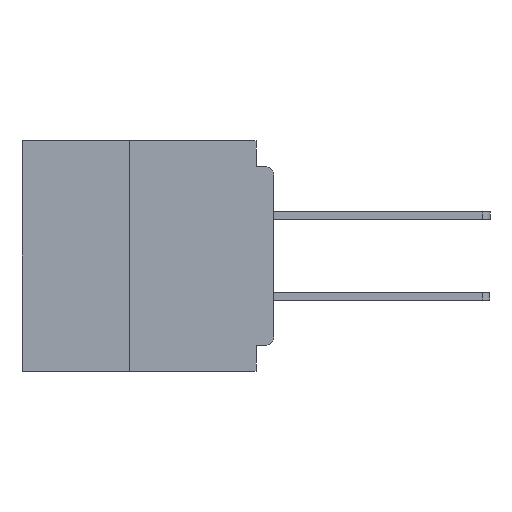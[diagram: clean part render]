
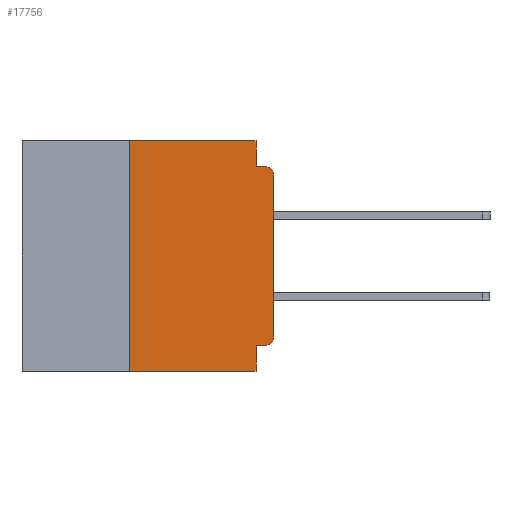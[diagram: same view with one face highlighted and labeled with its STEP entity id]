
A CAD part, left-side view. The second image highlights one B-rep face of the part: STEP entity #17756.
In plain terms, the highlighted planar face has unit normal (-1, 0, 0).
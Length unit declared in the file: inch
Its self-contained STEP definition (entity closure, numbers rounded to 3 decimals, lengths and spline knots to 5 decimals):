
#354 = DIRECTION ( 'NONE',  ( 0., 0., -1. ) ) ;
#1118 = EDGE_CURVE ( 'NONE', #3465, #8036, #11682, .T. ) ;
#2225 = CARTESIAN_POINT ( 'NONE',  ( 0., 0., -0.06 ) ) ;
#2336 = CARTESIAN_POINT ( 'NONE',  ( 0., 0.015, -0.355 ) ) ;
#2476 = EDGE_LOOP ( 'NONE', ( #45321, #27061, #30065, #25355, #29021, #8295, #48030, #5185, #6686, #10354 ) ) ;
#3120 = AXIS2_PLACEMENT_3D ( 'NONE', #16670, #45256, #20759 ) ;
#3465 = VERTEX_POINT ( 'NONE', #2336 ) ;
#3990 = CARTESIAN_POINT ( 'NONE',  ( 0., 0.031, 0. ) ) ;
#4482 = CARTESIAN_POINT ( 'NONE',  ( 0., 0.015, -0.045 ) ) ;
#4597 = CARTESIAN_POINT ( 'NONE',  ( 0., 0.031, -0.4 ) ) ;
#4685 = VERTEX_POINT ( 'NONE', #50907 ) ;
#5185 = ORIENTED_EDGE ( 'NONE', *, *, #27997, .F. ) ;
#5440 = CARTESIAN_POINT ( 'NONE',  ( 0., 0.031, -0.045 ) ) ;
#5860 = VERTEX_POINT ( 'NONE', #2225 ) ;
#5891 = FACE_OUTER_BOUND ( 'NONE', #2476, .T. ) ;
#6686 = ORIENTED_EDGE ( 'NONE', *, *, #1118, .F. ) ;
#7598 = VECTOR ( 'NONE', #35581, 39.37008 ) ;
#8036 = VERTEX_POINT ( 'NONE', #33725 ) ;
#8295 = ORIENTED_EDGE ( 'NONE', *, *, #31565, .F. ) ;
#9235 = VECTOR ( 'NONE', #28916, 39.37008 ) ;
#10112 = VERTEX_POINT ( 'NONE', #14600 ) ;
#10354 = ORIENTED_EDGE ( 'NONE', *, *, #42893, .T. ) ;
#10700 = PLANE ( 'NONE',  #35964 ) ;
#10829 = EDGE_CURVE ( 'NONE', #40173, #4685, #40249, .T. ) ;
#11139 = CARTESIAN_POINT ( 'NONE',  ( 0., 0.437, -0.4 ) ) ;
#11682 = LINE ( 'NONE', #42927, #12943 ) ;
#12357 = LINE ( 'NONE', #41577, #42395 ) ;
#12588 = VECTOR ( 'NONE', #354, 39.37008 ) ;
#12943 = VECTOR ( 'NONE', #42687, 39.37008 ) ;
#13446 = DIRECTION ( 'NONE',  ( 0., 0., -1. ) ) ;
#14117 = VECTOR ( 'NONE', #22977, 39.37008 ) ;
#14598 = DIRECTION ( 'NONE',  ( -1., 0., 0. ) ) ;
#14600 = CARTESIAN_POINT ( 'NONE',  ( 0., 0., -0.34 ) ) ;
#15902 = EDGE_CURVE ( 'NONE', #30779, #48542, #20163, .T. ) ;
#16670 = CARTESIAN_POINT ( 'NONE',  ( 0., 0.015, -0.06 ) ) ;
#17380 = CARTESIAN_POINT ( 'NONE',  ( 0., 0.437, 0. ) ) ;
#17605 = CIRCLE ( 'NONE', #3120, 0.015 ) ;
#17756 = ADVANCED_FACE ( 'NONE', ( #5891 ), #10700, .F. ) ;
#18917 = CARTESIAN_POINT ( 'NONE',  ( 0., 0., 0. ) ) ;
#18932 = CARTESIAN_POINT ( 'NONE',  ( 0., 0.437, 0. ) ) ;
#20163 = LINE ( 'NONE', #28741, #9235 ) ;
#20759 = DIRECTION ( 'NONE',  ( 0., 0., -1. ) ) ;
#21182 = DIRECTION ( 'NONE',  ( 0., 0., 1. ) ) ;
#22115 = EDGE_CURVE ( 'NONE', #10112, #5860, #25243, .T. ) ;
#22977 = DIRECTION ( 'NONE',  ( 0., 0., 1. ) ) ;
#22996 = DIRECTION ( 'NONE',  ( 0., 0., -1. ) ) ;
#23797 = VECTOR ( 'NONE', #29821, 39.37008 ) ;
#25243 = LINE ( 'NONE', #18917, #14117 ) ;
#25355 = ORIENTED_EDGE ( 'NONE', *, *, #30073, .F. ) ;
#25530 = CARTESIAN_POINT ( 'NONE',  ( 0., 0.031, 0. ) ) ;
#27061 = ORIENTED_EDGE ( 'NONE', *, *, #49108, .T. ) ;
#27997 = EDGE_CURVE ( 'NONE', #8036, #4685, #35566, .T. ) ;
#28741 = CARTESIAN_POINT ( 'NONE',  ( 0., 0., -0.045 ) ) ;
#28916 = DIRECTION ( 'NONE',  ( 0., -1., 0. ) ) ;
#29021 = ORIENTED_EDGE ( 'NONE', *, *, #35650, .F. ) ;
#29712 = VECTOR ( 'NONE', #13446, 39.37008 ) ;
#29821 = DIRECTION ( 'NONE',  ( 0., -1., 0. ) ) ;
#30065 = ORIENTED_EDGE ( 'NONE', *, *, #15902, .F. ) ;
#30073 = EDGE_CURVE ( 'NONE', #52705, #30779, #40642, .T. ) ;
#30779 = VERTEX_POINT ( 'NONE', #5440 ) ;
#31565 = EDGE_CURVE ( 'NONE', #40173, #34805, #12357, .T. ) ;
#31690 = CARTESIAN_POINT ( 'NONE',  ( 0., 0.25, -0.4 ) ) ;
#33725 = CARTESIAN_POINT ( 'NONE',  ( 0., 0.031, -0.355 ) ) ;
#34805 = VERTEX_POINT ( 'NONE', #44648 ) ;
#35566 = LINE ( 'NONE', #4597, #12588 ) ;
#35581 = DIRECTION ( 'NONE',  ( 0., -1., 0. ) ) ;
#35650 = EDGE_CURVE ( 'NONE', #34805, #52705, #37236, .T. ) ;
#35964 = AXIS2_PLACEMENT_3D ( 'NONE', #18932, #47523, #22996 ) ;
#37236 = LINE ( 'NONE', #17380, #23797 ) ;
#38382 = CIRCLE ( 'NONE', #43067, 0.015 ) ;
#39045 = CARTESIAN_POINT ( 'NONE',  ( 0., 0.015, -0.34 ) ) ;
#40173 = VERTEX_POINT ( 'NONE', #31690 ) ;
#40249 = LINE ( 'NONE', #11139, #7598 ) ;
#40642 = LINE ( 'NONE', #25530, #29712 ) ;
#41577 = CARTESIAN_POINT ( 'NONE',  ( 0., 0.25, -0.4 ) ) ;
#42395 = VECTOR ( 'NONE', #21182, 39.37008 ) ;
#42687 = DIRECTION ( 'NONE',  ( 0., 1., 0. ) ) ;
#42893 = EDGE_CURVE ( 'NONE', #3465, #10112, #38382, .T. ) ;
#42927 = CARTESIAN_POINT ( 'NONE',  ( 0., 0., -0.355 ) ) ;
#43067 = AXIS2_PLACEMENT_3D ( 'NONE', #39045, #14598, #43196 ) ;
#43196 = DIRECTION ( 'NONE',  ( 0., 0., -1. ) ) ;
#44648 = CARTESIAN_POINT ( 'NONE',  ( 0., 0.25, 0. ) ) ;
#45256 = DIRECTION ( 'NONE',  ( -1., 0., 0. ) ) ;
#45321 = ORIENTED_EDGE ( 'NONE', *, *, #22115, .T. ) ;
#47523 = DIRECTION ( 'NONE',  ( 1., 0., 0. ) ) ;
#48030 = ORIENTED_EDGE ( 'NONE', *, *, #10829, .T. ) ;
#48542 = VERTEX_POINT ( 'NONE', #4482 ) ;
#49108 = EDGE_CURVE ( 'NONE', #5860, #48542, #17605, .T. ) ;
#50907 = CARTESIAN_POINT ( 'NONE',  ( 0., 0.031, -0.4 ) ) ;
#52705 = VERTEX_POINT ( 'NONE', #3990 ) ;
